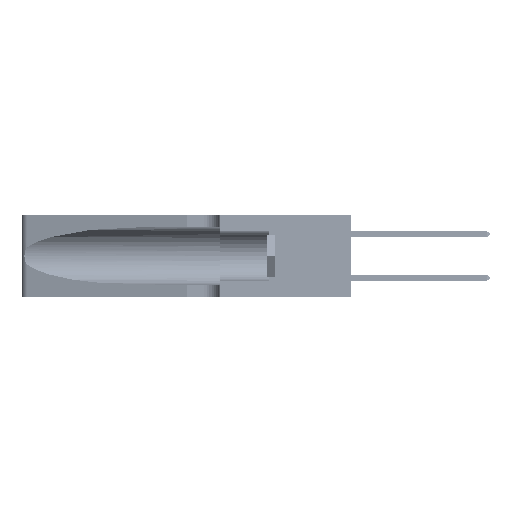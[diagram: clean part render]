
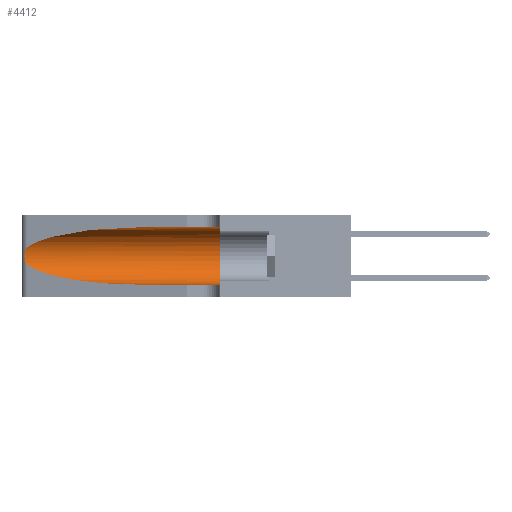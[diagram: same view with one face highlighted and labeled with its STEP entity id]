
A CAD part, left-side view. The second image highlights one B-rep face of the part: STEP entity #4412.
In plain terms, the highlighted cylindrical face has radius 3.308 mm (diameter 6.617 mm), a partial arc.
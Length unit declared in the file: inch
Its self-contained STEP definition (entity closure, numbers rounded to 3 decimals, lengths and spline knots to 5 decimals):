
#343 = CARTESIAN_POINT ( 'NONE',  ( 0.25487, 1.22718, 0.14631 ) ) ;
#2606 = CARTESIAN_POINT ( 'NONE',  ( 0.26075, 1.23896, 0.178 ) ) ;
#2879 = CARTESIAN_POINT ( 'NONE',  ( 0.1305, 0.35, 0.31525 ) ) ;
#4412 = ADVANCED_FACE ( 'NONE', ( #47787 ), #45147, .F. ) ;
#4415 = CARTESIAN_POINT ( 'NONE',  ( 0.25487, 1.22718, 0.14631 ) ) ;
#5551 = ORIENTED_EDGE ( 'NONE', *, *, #52513, .F. ) ;
#6434 = CARTESIAN_POINT ( 'NONE',  ( 0.2373, 1.15595, 0.28018 ) ) ;
#6936 = CARTESIAN_POINT ( 'NONE',  ( 0.25856, 1.23593, 0.16098 ) ) ;
#9893 = VECTOR ( 'NONE', #37669, 39.37008 ) ;
#11175 = CARTESIAN_POINT ( 'NONE',  ( 0.25639, 1.23186, 0.15144 ) ) ;
#11203 = LINE ( 'NONE', #25055, #9893 ) ;
#11592 = EDGE_CURVE ( 'NONE', #38736, #42255, #39986, .T. ) ;
#13641 = CARTESIAN_POINT ( 'NONE',  ( 0.1305, 1.61858, 0.185 ) ) ;
#15515 = CARTESIAN_POINT ( 'NONE',  ( 0.25487, 1.22718, 0.14631 ) ) ;
#15638 = ORIENTED_EDGE ( 'NONE', *, *, #26559, .T. ) ;
#16819 = ORIENTED_EDGE ( 'NONE', *, *, #18886, .F. ) ;
#17376 = CARTESIAN_POINT ( 'NONE',  ( 0.18966, 0.96281, 0.05475 ) ) ;
#18879 = ORIENTED_EDGE ( 'NONE', *, *, #48477, .T. ) ;
#18886 = EDGE_CURVE ( 'NONE', #37387, #33939, #53315, .T. ) ;
#19593 = CARTESIAN_POINT ( 'NONE',  ( 0.25639, 1.23184, 0.21858 ) ) ;
#21020 = EDGE_LOOP ( 'NONE', ( #21627, #18879, #45716, #15638, #16819, #5551 ) ) ;
#21502 = DIRECTION ( 'NONE',  ( 0., 1., 0. ) ) ;
#21607 = CARTESIAN_POINT ( 'NONE',  ( 0.2373, 1.15595, 0.08982 ) ) ;
#21627 = ORIENTED_EDGE ( 'NONE', *, *, #47835, .T. ) ;
#21673 = CARTESIAN_POINT ( 'NONE',  ( 0.1305, 0.35, 0.05475 ) ) ;
#22189 = DIRECTION ( 'NONE',  ( 0., -1., 0. ) ) ;
#23833 = CARTESIAN_POINT ( 'NONE',  ( 0.25854, 1.2359, 0.20912 ) ) ;
#24869 = LINE ( 'NONE', #25239, #48406 ) ;
#25055 = CARTESIAN_POINT ( 'NONE',  ( 0.1305, 1.61858, 0.31525 ) ) ;
#25239 = CARTESIAN_POINT ( 'NONE',  ( 0.1305, 1.61858, 0.05475 ) ) ;
#26275 = B_SPLINE_CURVE_WITH_KNOTS ( 'NONE', 3,
 ( #48688, #36260, #19593, #48875, #23833, #53112, #28033, #2606, #32251, #6936, #36437, #11175, #40632, #15515 ),
 .UNSPECIFIED., .F., .F.,
 ( 4, 2, 2, 2, 2, 2, 4 ),
 ( 0., 0.00027, 0.00053, 0.00107, 0.0016, 0.00187, 0.00214 ),
 .UNSPECIFIED. ) ;
#26559 = EDGE_CURVE ( 'NONE', #42255, #33939, #24869, .T. ) ;
#27319 = CARTESIAN_POINT ( 'NONE',  ( 0.25487, 1.22718, 0.22369 ) ) ;
#28033 = CARTESIAN_POINT ( 'NONE',  ( 0.26075, 1.23896, 0.19203 ) ) ;
#29457 = DIRECTION ( 'NONE',  ( 0., -1., 0. ) ) ;
#29751 = CARTESIAN_POINT ( 'NONE',  ( 0.1305, 0.72297, 0.31525 ) ) ;
#30037 = CARTESIAN_POINT ( 'NONE',  ( 0.1305, 0.72297, 0.05475 ) ) ;
#32251 = CARTESIAN_POINT ( 'NONE',  ( 0.26017, 1.23833, 0.17102 ) ) ;
#32906 = AXIS2_PLACEMENT_3D ( 'NONE', #46569, #21502, #50820 ) ;
#33900 = VERTEX_POINT ( 'NONE', #29751 ) ;
#33939 = VERTEX_POINT ( 'NONE', #21673 ) ;
#34589 = CARTESIAN_POINT ( 'NONE',  ( 0.1305, 0.72297, 0.05475 ) ) ;
#35935 = CARTESIAN_POINT ( 'NONE',  ( 0.25487, 1.22718, 0.22369 ) ) ;
#35977 =( BOUNDED_CURVE ( )  B_SPLINE_CURVE ( 3, ( #47415, #38998, #6434, #35935 ),
 .UNSPECIFIED., .F., .F. ) 
 B_SPLINE_CURVE_WITH_KNOTS ( ( 4, 4 ),
 ( 1.5708, 2.84003 ),
 .UNSPECIFIED. ) 
 CURVE ( )  GEOMETRIC_REPRESENTATION_ITEM ( )  RATIONAL_B_SPLINE_CURVE ( ( 1., 0.87, 0.87, 1. ) ) 
 REPRESENTATION_ITEM ( '' )  );
#36260 = CARTESIAN_POINT ( 'NONE',  ( 0.25555, 1.22994, 0.2215 ) ) ;
#36437 = CARTESIAN_POINT ( 'NONE',  ( 0.25789, 1.23486, 0.15765 ) ) ;
#37387 = VERTEX_POINT ( 'NONE', #2879 ) ;
#37669 = DIRECTION ( 'NONE',  ( 0., -1., 0. ) ) ;
#38736 = VERTEX_POINT ( 'NONE', #4415 ) ;
#38998 = CARTESIAN_POINT ( 'NONE',  ( 0.18966, 0.96281, 0.31525 ) ) ;
#39986 =( BOUNDED_CURVE ( )  B_SPLINE_CURVE ( 3, ( #343, #21607, #17376, #30037 ),
 .UNSPECIFIED., .F., .F. ) 
 B_SPLINE_CURVE_WITH_KNOTS ( ( 4, 4 ),
 ( 3.44316, 4.71239 ),
 .UNSPECIFIED. ) 
 CURVE ( )  GEOMETRIC_REPRESENTATION_ITEM ( )  RATIONAL_B_SPLINE_CURVE ( ( 1., 0.87, 0.87, 1. ) ) 
 REPRESENTATION_ITEM ( '' )  );
#40632 = CARTESIAN_POINT ( 'NONE',  ( 0.25555, 1.22993, 0.14849 ) ) ;
#42255 = VERTEX_POINT ( 'NONE', #34589 ) ;
#45147 = CYLINDRICAL_SURFACE ( 'NONE', #52267, 0.13025 ) ;
#45716 = ORIENTED_EDGE ( 'NONE', *, *, #11592, .T. ) ;
#46569 = CARTESIAN_POINT ( 'NONE',  ( 0.1305, 0.35, 0.185 ) ) ;
#47415 = CARTESIAN_POINT ( 'NONE',  ( 0.1305, 0.72297, 0.31525 ) ) ;
#47787 = FACE_OUTER_BOUND ( 'NONE', #21020, .T. ) ;
#47835 = EDGE_CURVE ( 'NONE', #33900, #50383, #35977, .T. ) ;
#48406 = VECTOR ( 'NONE', #29457, 39.37008 ) ;
#48477 = EDGE_CURVE ( 'NONE', #50383, #38736, #26275, .T. ) ;
#48688 = CARTESIAN_POINT ( 'NONE',  ( 0.25487, 1.22718, 0.22369 ) ) ;
#48875 = CARTESIAN_POINT ( 'NONE',  ( 0.25787, 1.23484, 0.2124 ) ) ;
#50383 = VERTEX_POINT ( 'NONE', #27319 ) ;
#50820 = DIRECTION ( 'NONE',  ( 0., 0., 1. ) ) ;
#51503 = DIRECTION ( 'NONE',  ( 0., 0., -1. ) ) ;
#52267 = AXIS2_PLACEMENT_3D ( 'NONE', #13641, #22189, #51503 ) ;
#52513 = EDGE_CURVE ( 'NONE', #33900, #37387, #11203, .T. ) ;
#53112 = CARTESIAN_POINT ( 'NONE',  ( 0.26018, 1.23835, 0.19895 ) ) ;
#53315 = CIRCLE ( 'NONE', #32906, 0.13025 ) ;
